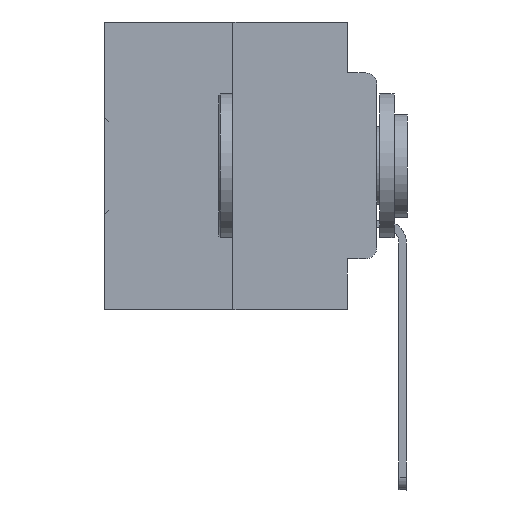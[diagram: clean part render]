
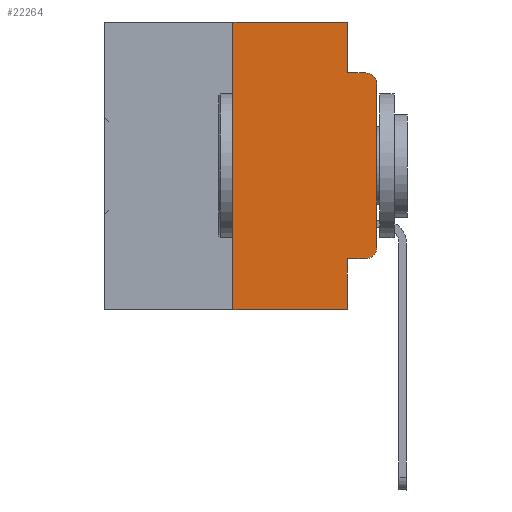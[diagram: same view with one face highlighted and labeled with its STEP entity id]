
A CAD part, left-side view. The second image highlights one B-rep face of the part: STEP entity #22264.
In plain terms, the highlighted planar face has unit normal (-1, 0, 0).
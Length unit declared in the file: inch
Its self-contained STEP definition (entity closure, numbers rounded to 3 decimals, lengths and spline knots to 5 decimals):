
#183 = DIRECTION ( 'NONE',  ( 0., -1., 0. ) ) ;
#373 = LINE ( 'NONE', #28205, #4598 ) ;
#1768 = CARTESIAN_POINT ( 'NONE',  ( 0., 0.02, -0.0885 ) ) ;
#2187 = ORIENTED_EDGE ( 'NONE', *, *, #2617, .F. ) ;
#2332 = CARTESIAN_POINT ( 'NONE',  ( 0., 0.051, -0.0885 ) ) ;
#2492 = VERTEX_POINT ( 'NONE', #36046 ) ;
#2617 = EDGE_CURVE ( 'NONE', #26529, #14279, #12738, .T. ) ;
#3458 = EDGE_CURVE ( 'NONE', #22064, #26529, #20421, .T. ) ;
#3923 = LINE ( 'NONE', #17394, #10583 ) ;
#4577 = ORIENTED_EDGE ( 'NONE', *, *, #15034, .T. ) ;
#4598 = VECTOR ( 'NONE', #183, 39.37008 ) ;
#5071 = DIRECTION ( 'NONE',  ( 0., 0., 1. ) ) ;
#5268 = ORIENTED_EDGE ( 'NONE', *, *, #8454, .F. ) ;
#5447 = CARTESIAN_POINT ( 'NONE',  ( 0., 0.25, 0. ) ) ;
#6098 = CARTESIAN_POINT ( 'NONE',  ( 0., 0.051, -0.4115 ) ) ;
#6127 = DIRECTION ( 'NONE',  ( 0., 0., -1. ) ) ;
#6835 = DIRECTION ( 'NONE',  ( 0., -1., 0. ) ) ;
#7288 = CIRCLE ( 'NONE', #32635, 0.02 ) ;
#7309 = CARTESIAN_POINT ( 'NONE',  ( 0., 0.473, 0. ) ) ;
#7529 = CARTESIAN_POINT ( 'NONE',  ( 0., 0.02, -0.3915 ) ) ;
#7907 = ORIENTED_EDGE ( 'NONE', *, *, #10334, .F. ) ;
#7968 = DIRECTION ( 'NONE',  ( 0., -1., 0. ) ) ;
#8224 = CARTESIAN_POINT ( 'NONE',  ( 0., 0.051, -0.4115 ) ) ;
#8333 = CARTESIAN_POINT ( 'NONE',  ( 0., 0.051, 0. ) ) ;
#8454 = EDGE_CURVE ( 'NONE', #31575, #22064, #373, .T. ) ;
#8488 = VERTEX_POINT ( 'NONE', #19920 ) ;
#10334 = EDGE_CURVE ( 'NONE', #2492, #31575, #3923, .T. ) ;
#10583 = VECTOR ( 'NONE', #34370, 39.37008 ) ;
#10722 = DIRECTION ( 'NONE',  ( 0., 0., -1. ) ) ;
#10837 = VECTOR ( 'NONE', #7968, 39.37008 ) ;
#10851 = ORIENTED_EDGE ( 'NONE', *, *, #34295, .T. ) ;
#12190 = CARTESIAN_POINT ( 'NONE',  ( 0., 0.051, -0.0885 ) ) ;
#12281 = DIRECTION ( 'NONE',  ( 0., 0., -1. ) ) ;
#12738 = LINE ( 'NONE', #12190, #24306 ) ;
#13497 = CARTESIAN_POINT ( 'NONE',  ( 0., 0.02, -0.1085 ) ) ;
#13549 = CARTESIAN_POINT ( 'NONE',  ( 0., 0., -0.3915 ) ) ;
#13678 = CARTESIAN_POINT ( 'NONE',  ( 0., 0.473, -0.5 ) ) ;
#14250 = VECTOR ( 'NONE', #6127, 39.37008 ) ;
#14277 = ORIENTED_EDGE ( 'NONE', *, *, #17354, .T. ) ;
#14279 = VERTEX_POINT ( 'NONE', #1768 ) ;
#14309 = VECTOR ( 'NONE', #25816, 39.37008 ) ;
#15034 = EDGE_CURVE ( 'NONE', #15608, #35134, #31356, .T. ) ;
#15608 = VERTEX_POINT ( 'NONE', #8224 ) ;
#16667 = AXIS2_PLACEMENT_3D ( 'NONE', #7309, #18575, #18032 ) ;
#16839 = AXIS2_PLACEMENT_3D ( 'NONE', #7529, #21732, #27255 ) ;
#17276 = CARTESIAN_POINT ( 'NONE',  ( 0., 0.051, 0. ) ) ;
#17354 = EDGE_CURVE ( 'NONE', #28217, #31474, #27733, .T. ) ;
#17394 = CARTESIAN_POINT ( 'NONE',  ( 0., 0.25, 0. ) ) ;
#17589 = ORIENTED_EDGE ( 'NONE', *, *, #24550, .T. ) ;
#18032 = DIRECTION ( 'NONE',  ( 0., 0., -1. ) ) ;
#18575 = DIRECTION ( 'NONE',  ( 1., 0., 0. ) ) ;
#19538 = ORIENTED_EDGE ( 'NONE', *, *, #24596, .T. ) ;
#19741 = VECTOR ( 'NONE', #5071, 39.37008 ) ;
#19920 = CARTESIAN_POINT ( 'NONE',  ( 0., 0.051, -0.5 ) ) ;
#20421 = LINE ( 'NONE', #17276, #35915 ) ;
#21184 = EDGE_CURVE ( 'NONE', #15608, #8488, #34169, .T. ) ;
#21732 = DIRECTION ( 'NONE',  ( -1., 0., 0. ) ) ;
#21836 = CARTESIAN_POINT ( 'NONE',  ( 0., 0., 0. ) ) ;
#22064 = VERTEX_POINT ( 'NONE', #32204 ) ;
#22264 = ADVANCED_FACE ( 'NONE', ( #32235 ), #24270, .F. ) ;
#23328 = CARTESIAN_POINT ( 'NONE',  ( 0., 0.02, -0.4115 ) ) ;
#23500 = EDGE_LOOP ( 'NONE', ( #14277, #19538, #2187, #31430, #5268, #7907, #17589, #27768, #4577, #10851 ) ) ;
#23905 = CARTESIAN_POINT ( 'NONE',  ( 0., 0., -0.1085 ) ) ;
#24270 = PLANE ( 'NONE',  #16667 ) ;
#24306 = VECTOR ( 'NONE', #6835, 39.37008 ) ;
#24550 = EDGE_CURVE ( 'NONE', #2492, #8488, #27510, .T. ) ;
#24596 = EDGE_CURVE ( 'NONE', #31474, #14279, #7288, .T. ) ;
#24728 = DIRECTION ( 'NONE',  ( -1., 0., 0. ) ) ;
#25816 = DIRECTION ( 'NONE',  ( 0., -1., 0. ) ) ;
#26529 = VERTEX_POINT ( 'NONE', #2332 ) ;
#27255 = DIRECTION ( 'NONE',  ( 0., 0., -1. ) ) ;
#27510 = LINE ( 'NONE', #13678, #10837 ) ;
#27733 = LINE ( 'NONE', #21836, #19741 ) ;
#27768 = ORIENTED_EDGE ( 'NONE', *, *, #21184, .F. ) ;
#28205 = CARTESIAN_POINT ( 'NONE',  ( 0., 0.473, 0. ) ) ;
#28217 = VERTEX_POINT ( 'NONE', #13549 ) ;
#31356 = LINE ( 'NONE', #6098, #14309 ) ;
#31430 = ORIENTED_EDGE ( 'NONE', *, *, #3458, .F. ) ;
#31474 = VERTEX_POINT ( 'NONE', #23905 ) ;
#31575 = VERTEX_POINT ( 'NONE', #5447 ) ;
#32204 = CARTESIAN_POINT ( 'NONE',  ( 0., 0.051, 0. ) ) ;
#32235 = FACE_OUTER_BOUND ( 'NONE', #23500, .T. ) ;
#32635 = AXIS2_PLACEMENT_3D ( 'NONE', #13497, #24728, #10722 ) ;
#33346 = CIRCLE ( 'NONE', #16839, 0.02 ) ;
#34169 = LINE ( 'NONE', #8333, #14250 ) ;
#34295 = EDGE_CURVE ( 'NONE', #35134, #28217, #33346, .T. ) ;
#34370 = DIRECTION ( 'NONE',  ( 0., 0., 1. ) ) ;
#35134 = VERTEX_POINT ( 'NONE', #23328 ) ;
#35915 = VECTOR ( 'NONE', #12281, 39.37008 ) ;
#36046 = CARTESIAN_POINT ( 'NONE',  ( 0., 0.25, -0.5 ) ) ;
